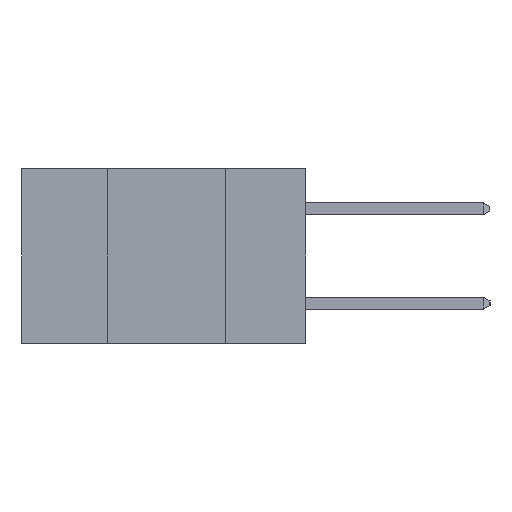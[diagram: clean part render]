
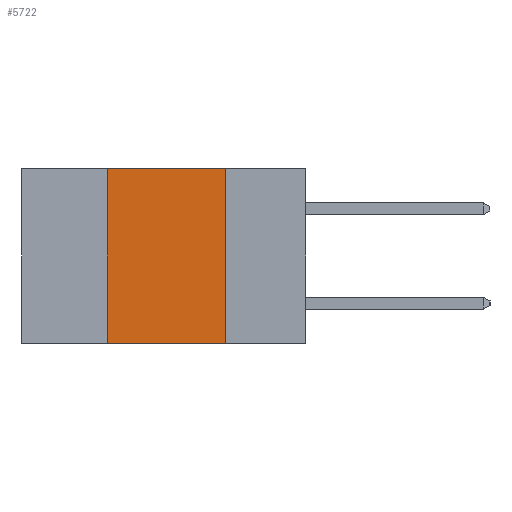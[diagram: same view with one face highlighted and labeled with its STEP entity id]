
A CAD part, left-side view. The second image highlights one B-rep face of the part: STEP entity #5722.
In plain terms, the highlighted planar face has unit normal (-1, 0, 0).
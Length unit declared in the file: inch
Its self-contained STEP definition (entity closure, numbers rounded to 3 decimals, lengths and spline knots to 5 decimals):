
#680 = ORIENTED_EDGE ( 'NONE', *, *, #4083, .T. ) ;
#1212 = DIRECTION ( 'NONE',  ( 0., 0., -1. ) ) ;
#1458 = DIRECTION ( 'NONE',  ( 1., 0., 0. ) ) ;
#1799 = DIRECTION ( 'NONE',  ( 0., 0., -1. ) ) ;
#1813 = CARTESIAN_POINT ( 'NONE',  ( 0., 0.17, -0.37 ) ) ;
#1895 = CARTESIAN_POINT ( 'NONE',  ( 0., 0.17, -0.37 ) ) ;
#2690 = PLANE ( 'NONE',  #16596 ) ;
#3420 = CARTESIAN_POINT ( 'NONE',  ( 0., 0.6, 0. ) ) ;
#3619 = CARTESIAN_POINT ( 'NONE',  ( 0., 0.42, -0.37 ) ) ;
#4083 = EDGE_CURVE ( 'NONE', #5707, #20715, #10810, .T. ) ;
#4335 = VECTOR ( 'NONE', #1212, 39.37008 ) ;
#5335 = VERTEX_POINT ( 'NONE', #8907 ) ;
#5411 = CARTESIAN_POINT ( 'NONE',  ( 0., 0.6, -0.37 ) ) ;
#5462 = FACE_OUTER_BOUND ( 'NONE', #20729, .T. ) ;
#5570 = DIRECTION ( 'NONE',  ( 0., -1., 0. ) ) ;
#5603 = VECTOR ( 'NONE', #7388, 39.37008 ) ;
#5707 = VERTEX_POINT ( 'NONE', #3619 ) ;
#5722 = ADVANCED_FACE ( 'NONE', ( #5462 ), #2690, .F. ) ;
#6676 = EDGE_CURVE ( 'NONE', #17956, #20715, #8850, .T. ) ;
#7141 = DIRECTION ( 'NONE',  ( 0., 0., 1. ) ) ;
#7388 = DIRECTION ( 'NONE',  ( 0., -1., 0. ) ) ;
#8221 = EDGE_CURVE ( 'NONE', #5335, #17956, #10111, .T. ) ;
#8850 = LINE ( 'NONE', #1813, #4335 ) ;
#8907 = CARTESIAN_POINT ( 'NONE',  ( 0., 0.42, 0. ) ) ;
#8912 = LINE ( 'NONE', #18653, #21497 ) ;
#10111 = LINE ( 'NONE', #20489, #5603 ) ;
#10810 = LINE ( 'NONE', #5411, #18995 ) ;
#14213 = EDGE_CURVE ( 'NONE', #5707, #5335, #8912, .T. ) ;
#16596 = AXIS2_PLACEMENT_3D ( 'NONE', #3420, #1458, #1799 ) ;
#16880 = ORIENTED_EDGE ( 'NONE', *, *, #6676, .F. ) ;
#17378 = ORIENTED_EDGE ( 'NONE', *, *, #8221, .F. ) ;
#17873 = ORIENTED_EDGE ( 'NONE', *, *, #14213, .F. ) ;
#17956 = VERTEX_POINT ( 'NONE', #19436 ) ;
#18653 = CARTESIAN_POINT ( 'NONE',  ( 0., 0.42, -0.37 ) ) ;
#18995 = VECTOR ( 'NONE', #5570, 39.37008 ) ;
#19436 = CARTESIAN_POINT ( 'NONE',  ( 0., 0.17, 0. ) ) ;
#20489 = CARTESIAN_POINT ( 'NONE',  ( 0., 0.6, 0. ) ) ;
#20715 = VERTEX_POINT ( 'NONE', #1895 ) ;
#20729 = EDGE_LOOP ( 'NONE', ( #16880, #17378, #17873, #680 ) ) ;
#21497 = VECTOR ( 'NONE', #7141, 39.37008 ) ;
